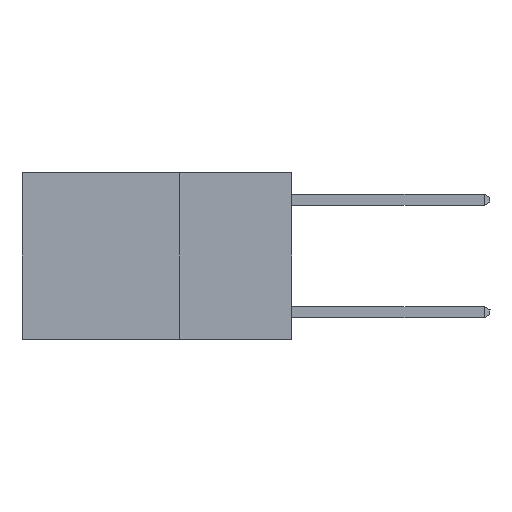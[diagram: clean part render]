
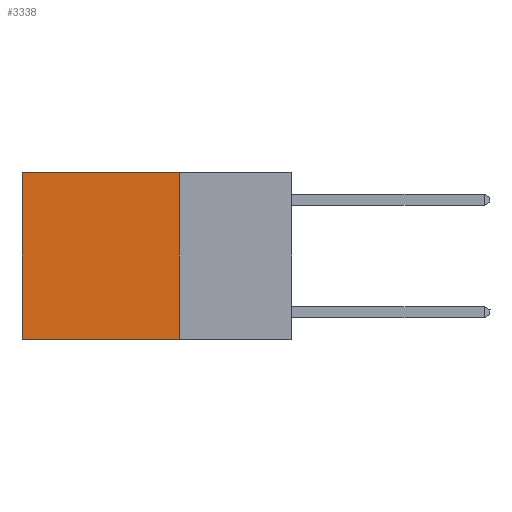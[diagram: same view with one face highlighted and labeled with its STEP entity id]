
A CAD part, left-side view. The second image highlights one B-rep face of the part: STEP entity #3338.
In plain terms, the highlighted planar face has unit normal (-1, 0, 0).
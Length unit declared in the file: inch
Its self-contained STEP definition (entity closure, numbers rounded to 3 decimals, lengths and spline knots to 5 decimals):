
#59 = LINE ( 'NONE', #7221, #8282 ) ;
#1279 = VECTOR ( 'NONE', #12296, 39.37008 ) ;
#1605 = LINE ( 'NONE', #12308, #1279 ) ;
#1916 = ORIENTED_EDGE ( 'NONE', *, *, #4552, .F. ) ;
#2121 = EDGE_CURVE ( 'NONE', #7294, #12074, #1605, .T. ) ;
#2350 = VERTEX_POINT ( 'NONE', #10524 ) ;
#2361 = LINE ( 'NONE', #8524, #8181 ) ;
#3226 = ORIENTED_EDGE ( 'NONE', *, *, #10625, .T. ) ;
#3338 = ADVANCED_FACE ( 'NONE', ( #11306 ), #13195, .F. ) ;
#4552 = EDGE_CURVE ( 'NONE', #11765, #2350, #9028, .T. ) ;
#5122 = ORIENTED_EDGE ( 'NONE', *, *, #13020, .F. ) ;
#6058 = ORIENTED_EDGE ( 'NONE', *, *, #2121, .T. ) ;
#6214 = CARTESIAN_POINT ( 'NONE',  ( 0.2625, 0.25, 0. ) ) ;
#6341 = AXIS2_PLACEMENT_3D ( 'NONE', #13184, #13157, #13154 ) ;
#7221 = CARTESIAN_POINT ( 'NONE',  ( 0.2625, 0.25, -0.37 ) ) ;
#7294 = VERTEX_POINT ( 'NONE', #12425 ) ;
#8181 = VECTOR ( 'NONE', #9491, 39.37008 ) ;
#8187 = CARTESIAN_POINT ( 'NONE',  ( 0.2625, 0.6, -0.37 ) ) ;
#8257 = DIRECTION ( 'NONE',  ( 0., 1., 0. ) ) ;
#8282 = VECTOR ( 'NONE', #8257, 39.37008 ) ;
#8524 = CARTESIAN_POINT ( 'NONE',  ( 0.2625, 0.25, 0. ) ) ;
#9028 = LINE ( 'NONE', #6214, #11656 ) ;
#9491 = DIRECTION ( 'NONE',  ( 0., 1., 0. ) ) ;
#9580 = EDGE_LOOP ( 'NONE', ( #6058, #5122, #1916, #3226 ) ) ;
#10524 = CARTESIAN_POINT ( 'NONE',  ( 0.2625, 0.25, -0.37 ) ) ;
#10625 = EDGE_CURVE ( 'NONE', #11765, #7294, #2361, .T. ) ;
#11306 = FACE_OUTER_BOUND ( 'NONE', #9580, .T. ) ;
#11656 = VECTOR ( 'NONE', #13230, 39.37008 ) ;
#11765 = VERTEX_POINT ( 'NONE', #12730 ) ;
#12074 = VERTEX_POINT ( 'NONE', #8187 ) ;
#12296 = DIRECTION ( 'NONE',  ( 0., 0., -1. ) ) ;
#12308 = CARTESIAN_POINT ( 'NONE',  ( 0.2625, 0.6, 0. ) ) ;
#12425 = CARTESIAN_POINT ( 'NONE',  ( 0.2625, 0.6, 0. ) ) ;
#12730 = CARTESIAN_POINT ( 'NONE',  ( 0.2625, 0.25, 0. ) ) ;
#13020 = EDGE_CURVE ( 'NONE', #2350, #12074, #59, .T. ) ;
#13154 = DIRECTION ( 'NONE',  ( 0., 0., -1. ) ) ;
#13157 = DIRECTION ( 'NONE',  ( 1., 0., 0. ) ) ;
#13184 = CARTESIAN_POINT ( 'NONE',  ( 0.2625, 0.25, 0. ) ) ;
#13195 = PLANE ( 'NONE',  #6341 ) ;
#13230 = DIRECTION ( 'NONE',  ( 0., 0., -1. ) ) ;
